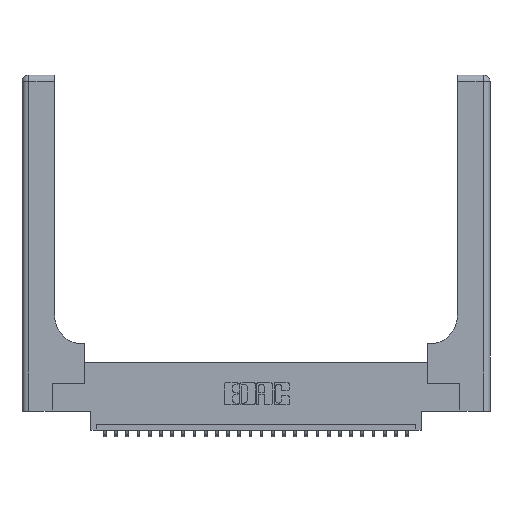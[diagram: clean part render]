
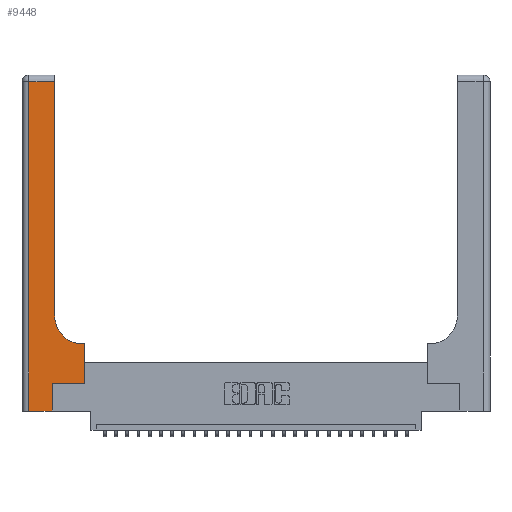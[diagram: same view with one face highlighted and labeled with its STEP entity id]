
A CAD part, top view. The second image highlights one B-rep face of the part: STEP entity #9448.
In plain terms, the highlighted planar face has unit normal (0, 0, 1).
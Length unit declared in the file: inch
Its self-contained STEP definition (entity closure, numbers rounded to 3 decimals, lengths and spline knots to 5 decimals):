
#82 = EDGE_CURVE ( 'NONE', #8329, #202, #8793, .T. ) ;
#202 = VERTEX_POINT ( 'NONE', #14082 ) ;
#244 = ORIENTED_EDGE ( 'NONE', *, *, #28209, .T. ) ;
#246 = ORIENTED_EDGE ( 'NONE', *, *, #5865, .T. ) ;
#814 = PLANE ( 'NONE',  #18623 ) ;
#821 = CARTESIAN_POINT ( 'NONE',  ( 0., 2.94, 0.37 ) ) ;
#1154 = ORIENTED_EDGE ( 'NONE', *, *, #23752, .T. ) ;
#1741 = DIRECTION ( 'NONE',  ( 0., 1., 0. ) ) ;
#3001 = VECTOR ( 'NONE', #3948, 39.37008 ) ;
#3255 = CARTESIAN_POINT ( 'NONE',  ( 0.269, 0., 0.37 ) ) ;
#3560 = LINE ( 'NONE', #7031, #26500 ) ;
#3948 = DIRECTION ( 'NONE',  ( 1., 0., 0. ) ) ;
#4078 = EDGE_CURVE ( 'NONE', #202, #5453, #20911, .T. ) ;
#4608 = CARTESIAN_POINT ( 'NONE',  ( 0.2915, 0.6, 0.37 ) ) ;
#4771 = FACE_OUTER_BOUND ( 'NONE', #23265, .T. ) ;
#4850 = CARTESIAN_POINT ( 'NONE',  ( 0.06, 0., 0.37 ) ) ;
#5288 = CARTESIAN_POINT ( 'NONE',  ( 0., 3., 0.37 ) ) ;
#5453 = VERTEX_POINT ( 'NONE', #20673 ) ;
#5865 = EDGE_CURVE ( 'NONE', #10524, #8329, #9074, .T. ) ;
#6218 = CARTESIAN_POINT ( 'NONE',  ( 0.269, 0.25, 0.37 ) ) ;
#6920 = CARTESIAN_POINT ( 'NONE',  ( 0.269, 0., 0.37 ) ) ;
#7031 = CARTESIAN_POINT ( 'NONE',  ( 0.06, 3., 0.37 ) ) ;
#7381 = LINE ( 'NONE', #6218, #26916 ) ;
#7562 = ORIENTED_EDGE ( 'NONE', *, *, #23365, .T. ) ;
#7699 = VECTOR ( 'NONE', #20620, 39.37008 ) ;
#8329 = VERTEX_POINT ( 'NONE', #8567 ) ;
#8567 = CARTESIAN_POINT ( 'NONE',  ( 0.5585, 0.6, 0.37 ) ) ;
#8793 = LINE ( 'NONE', #4608, #21140 ) ;
#9074 = LINE ( 'NONE', #12159, #17999 ) ;
#9448 = ADVANCED_FACE ( 'NONE', ( #4771 ), #814, .F. ) ;
#10120 = CARTESIAN_POINT ( 'NONE',  ( 0.2915, 3., 0.37 ) ) ;
#10440 = CARTESIAN_POINT ( 'NONE',  ( 0.2915, 2.94, 0.37 ) ) ;
#10508 = VECTOR ( 'NONE', #1741, 39.37008 ) ;
#10524 = VERTEX_POINT ( 'NONE', #26054 ) ;
#10542 = CARTESIAN_POINT ( 'NONE',  ( 0.5415, 0.85, 0.37 ) ) ;
#10687 = VERTEX_POINT ( 'NONE', #19614 ) ;
#11074 = EDGE_CURVE ( 'NONE', #16911, #15429, #25639, .T. ) ;
#11839 = VECTOR ( 'NONE', #20510, 39.37008 ) ;
#12159 = CARTESIAN_POINT ( 'NONE',  ( 0.5585, 0.25, 0.37 ) ) ;
#12163 = VERTEX_POINT ( 'NONE', #27840 ) ;
#12919 = DIRECTION ( 'NONE',  ( 1., 0., 0. ) ) ;
#13099 = ORIENTED_EDGE ( 'NONE', *, *, #82, .T. ) ;
#14082 = CARTESIAN_POINT ( 'NONE',  ( 0.5415, 0.6, 0.37 ) ) ;
#14517 = AXIS2_PLACEMENT_3D ( 'NONE', #10542, #25911, #28077 ) ;
#14663 = DIRECTION ( 'NONE',  ( -1., 0., 0. ) ) ;
#15429 = VERTEX_POINT ( 'NONE', #6920 ) ;
#15990 = ORIENTED_EDGE ( 'NONE', *, *, #18834, .T. ) ;
#16911 = VERTEX_POINT ( 'NONE', #4850 ) ;
#17174 = CARTESIAN_POINT ( 'NONE',  ( 0., 0., 0.37 ) ) ;
#17692 = LINE ( 'NONE', #821, #11839 ) ;
#17713 = LINE ( 'NONE', #10120, #10508 ) ;
#17999 = VECTOR ( 'NONE', #25394, 39.37008 ) ;
#18623 = AXIS2_PLACEMENT_3D ( 'NONE', #5288, #22747, #22943 ) ;
#18834 = EDGE_CURVE ( 'NONE', #12163, #16911, #3560, .T. ) ;
#19614 = CARTESIAN_POINT ( 'NONE',  ( 0.269, 0.25, 0.37 ) ) ;
#20510 = DIRECTION ( 'NONE',  ( -1., 0., 0. ) ) ;
#20620 = DIRECTION ( 'NONE',  ( 0., 1., 0. ) ) ;
#20673 = CARTESIAN_POINT ( 'NONE',  ( 0.2915, 0.85, 0.37 ) ) ;
#20911 = CIRCLE ( 'NONE', #14517, 0.25 ) ;
#21140 = VECTOR ( 'NONE', #14663, 39.37008 ) ;
#22204 = DIRECTION ( 'NONE',  ( 0., -1., 0. ) ) ;
#22747 = DIRECTION ( 'NONE',  ( 0., 0., -1. ) ) ;
#22904 = ORIENTED_EDGE ( 'NONE', *, *, #11074, .T. ) ;
#22943 = DIRECTION ( 'NONE',  ( -1., 0., 0. ) ) ;
#23189 = VERTEX_POINT ( 'NONE', #10440 ) ;
#23265 = EDGE_LOOP ( 'NONE', ( #244, #28150, #15990, #22904, #1154, #7562, #246, #13099, #25864 ) ) ;
#23365 = EDGE_CURVE ( 'NONE', #10687, #10524, #7381, .T. ) ;
#23674 = EDGE_CURVE ( 'NONE', #23189, #12163, #17692, .T. ) ;
#23752 = EDGE_CURVE ( 'NONE', #15429, #10687, #25215, .T. ) ;
#25215 = LINE ( 'NONE', #3255, #7699 ) ;
#25394 = DIRECTION ( 'NONE',  ( 0., 1., 0. ) ) ;
#25639 = LINE ( 'NONE', #17174, #3001 ) ;
#25864 = ORIENTED_EDGE ( 'NONE', *, *, #4078, .T. ) ;
#25911 = DIRECTION ( 'NONE',  ( 0., 0., -1. ) ) ;
#26054 = CARTESIAN_POINT ( 'NONE',  ( 0.5585, 0.25, 0.37 ) ) ;
#26500 = VECTOR ( 'NONE', #22204, 39.37008 ) ;
#26916 = VECTOR ( 'NONE', #12919, 39.37008 ) ;
#27840 = CARTESIAN_POINT ( 'NONE',  ( 0.06, 2.94, 0.37 ) ) ;
#28077 = DIRECTION ( 'NONE',  ( 1., 0., 0. ) ) ;
#28150 = ORIENTED_EDGE ( 'NONE', *, *, #23674, .T. ) ;
#28209 = EDGE_CURVE ( 'NONE', #5453, #23189, #17713, .T. ) ;
